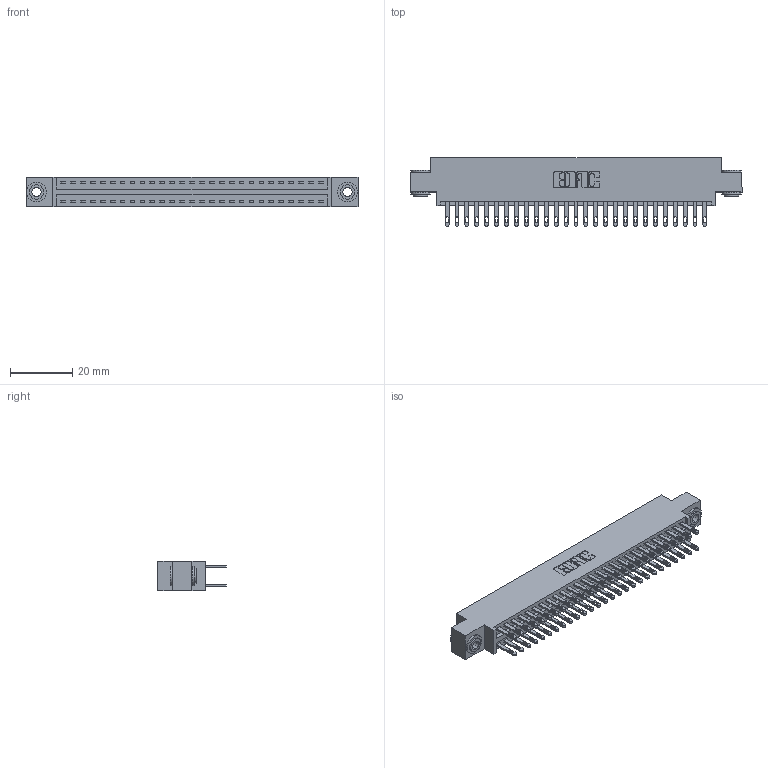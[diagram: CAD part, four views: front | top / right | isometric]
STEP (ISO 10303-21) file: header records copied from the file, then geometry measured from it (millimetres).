
FILE_DESCRIPTION (( 'STEP AP203' ), '1' );
FILE_NAME ('896-054-500-803.STEP', '2021-07-27T23:56:58', ( '' ), ( '' ), 'SwSTEP 2.0', 'SolidWorks 2020', '' );
FILE_SCHEMA (( 'CONFIG_CONTROL_DESIGN' ));
Length unit declared in the file: inch
Products named in the file (4): 896-054-500-803; 345-250-002_345-250-002-102; 345-292-001_345-293-100; 846 Part_0.170 Offset - 0.156 Dia-TH
Assembly tree (57 placements, depth 2):
  896-054-500-803
    846 Part_0.170 Offset - 0.156 Dia-TH
    345-292-001_345-293-100  x54
    345-250-002_345-250-002-102  x2
Bounding box: 106.3 x 21.84 x 9.4 mm (x, y, z)
Volume: 10278.8 mm3; surface area: 14852.1 mm2
Topology: 57 solids, 57 shells, 2756 faces, 8355 edges, 5566 vertices
Faces by surface type: plane 1656, cylinder 1092, cone 8
Entity records: 20352 total; most frequent: CARTESIAN_POINT 3351, ORIENTED_EDGE 3278, DIRECTION 3037, EDGE_CURVE 1639, LINE 1371, VECTOR 1371, VERTEX_POINT 1090, AXIS2_PLACEMENT_3D 833
